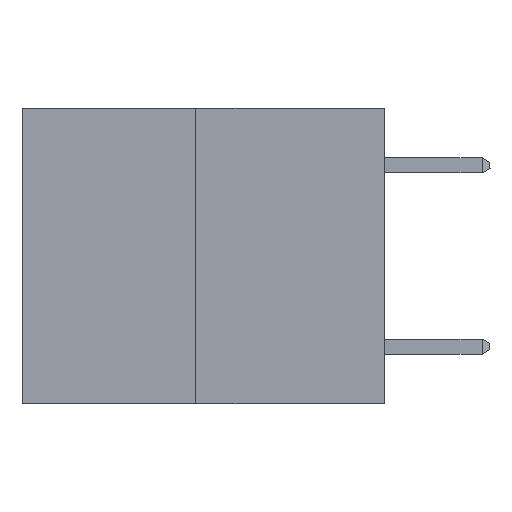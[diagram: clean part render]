
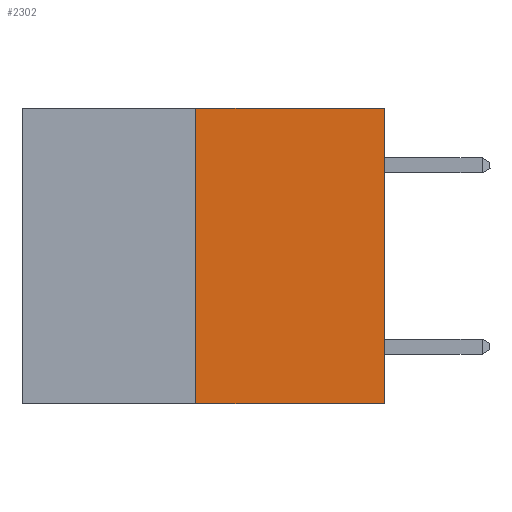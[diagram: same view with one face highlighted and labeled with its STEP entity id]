
A CAD part, left-side view. The second image highlights one B-rep face of the part: STEP entity #2302.
In plain terms, the highlighted planar face has unit normal (-1, 0, 0).
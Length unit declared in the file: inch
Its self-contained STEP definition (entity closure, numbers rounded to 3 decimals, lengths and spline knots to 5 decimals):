
#760 = CARTESIAN_POINT ( 'NONE',  ( 0., 0.312, -0.49 ) ) ;
#1792 = DIRECTION ( 'NONE',  ( 0., 0., 1. ) ) ;
#2302 = ADVANCED_FACE ( 'NONE', ( #26621 ), #4781, .F. ) ;
#2436 = LINE ( 'NONE', #29776, #12141 ) ;
#2921 = EDGE_CURVE ( 'NONE', #24582, #7530, #20324, .T. ) ;
#3314 = EDGE_CURVE ( 'NONE', #11881, #7530, #2436, .T. ) ;
#3673 = EDGE_CURVE ( 'NONE', #12852, #24582, #11745, .T. ) ;
#3936 = ORIENTED_EDGE ( 'NONE', *, *, #2921, .T. ) ;
#4193 = ORIENTED_EDGE ( 'NONE', *, *, #3673, .T. ) ;
#4781 = PLANE ( 'NONE',  #11438 ) ;
#6166 = CARTESIAN_POINT ( 'NONE',  ( 0., 0., 0. ) ) ;
#7284 = CARTESIAN_POINT ( 'NONE',  ( 0., 0.6, 0. ) ) ;
#7530 = VERTEX_POINT ( 'NONE', #6166 ) ;
#7671 = LINE ( 'NONE', #760, #12516 ) ;
#8133 = CARTESIAN_POINT ( 'NONE',  ( 0., 0., -0.49 ) ) ;
#9892 = CARTESIAN_POINT ( 'NONE',  ( 0., 0.6, -0.49 ) ) ;
#10251 = VECTOR ( 'NONE', #14499, 39.37008 ) ;
#11438 = AXIS2_PLACEMENT_3D ( 'NONE', #7284, #21089, #27518 ) ;
#11745 = LINE ( 'NONE', #9892, #10251 ) ;
#11881 = VERTEX_POINT ( 'NONE', #13925 ) ;
#12062 = EDGE_LOOP ( 'NONE', ( #20004, #4193, #3936, #22904 ) ) ;
#12141 = VECTOR ( 'NONE', #27286, 39.37008 ) ;
#12516 = VECTOR ( 'NONE', #19974, 39.37008 ) ;
#12852 = VERTEX_POINT ( 'NONE', #16795 ) ;
#13241 = EDGE_CURVE ( 'NONE', #12852, #11881, #7671, .T. ) ;
#13925 = CARTESIAN_POINT ( 'NONE',  ( 0., 0.312, 0. ) ) ;
#14499 = DIRECTION ( 'NONE',  ( 0., -1., 0. ) ) ;
#16795 = CARTESIAN_POINT ( 'NONE',  ( 0., 0.312, -0.49 ) ) ;
#19974 = DIRECTION ( 'NONE',  ( 0., 0., 1. ) ) ;
#20004 = ORIENTED_EDGE ( 'NONE', *, *, #13241, .F. ) ;
#20324 = LINE ( 'NONE', #27787, #23306 ) ;
#21089 = DIRECTION ( 'NONE',  ( 1., 0., 0. ) ) ;
#22904 = ORIENTED_EDGE ( 'NONE', *, *, #3314, .F. ) ;
#23306 = VECTOR ( 'NONE', #1792, 39.37008 ) ;
#24582 = VERTEX_POINT ( 'NONE', #8133 ) ;
#26621 = FACE_OUTER_BOUND ( 'NONE', #12062, .T. ) ;
#27286 = DIRECTION ( 'NONE',  ( 0., -1., 0. ) ) ;
#27518 = DIRECTION ( 'NONE',  ( 0., 0., -1. ) ) ;
#27787 = CARTESIAN_POINT ( 'NONE',  ( 0., 0., 0. ) ) ;
#29776 = CARTESIAN_POINT ( 'NONE',  ( 0., 0.6, 0. ) ) ;
